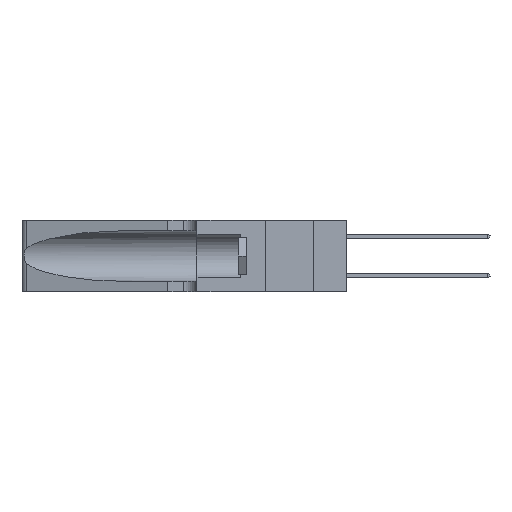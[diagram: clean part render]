
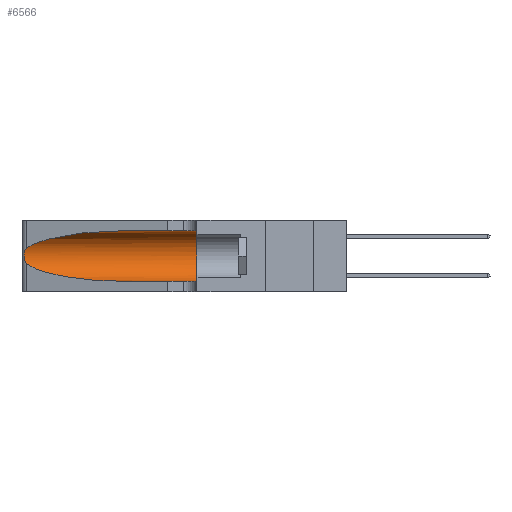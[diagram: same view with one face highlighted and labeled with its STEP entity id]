
A CAD part, left-side view. The second image highlights one B-rep face of the part: STEP entity #6566.
In plain terms, the highlighted cylindrical face has radius 3.308 mm (diameter 6.617 mm), a partial arc.
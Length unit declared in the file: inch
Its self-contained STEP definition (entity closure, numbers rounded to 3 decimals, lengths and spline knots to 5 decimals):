
#51 = VERTEX_POINT ( 'NONE', #33860 ) ;
#889 =( BOUNDED_CURVE ( )  B_SPLINE_CURVE ( 3, ( #27902, #6060, #30596, #14412 ),
 .UNSPECIFIED., .F., .F. ) 
 B_SPLINE_CURVE_WITH_KNOTS ( ( 4, 4 ),
 ( 3.44316, 4.71239 ),
 .UNSPECIFIED. ) 
 CURVE ( )  GEOMETRIC_REPRESENTATION_ITEM ( )  RATIONAL_B_SPLINE_CURVE ( ( 1., 0.87, 0.87, 1. ) ) 
 REPRESENTATION_ITEM ( '' )  );
#1834 = CARTESIAN_POINT ( 'NONE',  ( 0.1305, 0.35, 0.185 ) ) ;
#2090 = VERTEX_POINT ( 'NONE', #12327 ) ;
#2683 = CARTESIAN_POINT ( 'NONE',  ( 0.25789, 1.23486, 0.15765 ) ) ;
#3018 = VERTEX_POINT ( 'NONE', #10721 ) ;
#3440 = AXIS2_PLACEMENT_3D ( 'NONE', #1834, #20915, #4614 ) ;
#4614 = DIRECTION ( 'NONE',  ( 0., 0., 1. ) ) ;
#4886 = VERTEX_POINT ( 'NONE', #28967 ) ;
#4904 = DIRECTION ( 'NONE',  ( 0., -1., 0. ) ) ;
#5040 = CARTESIAN_POINT ( 'NONE',  ( 0.1305, 1.61858, 0.185 ) ) ;
#5468 = CARTESIAN_POINT ( 'NONE',  ( 0.25555, 1.22993, 0.14849 ) ) ;
#5615 = ORIENTED_EDGE ( 'NONE', *, *, #15021, .F. ) ;
#6060 = CARTESIAN_POINT ( 'NONE',  ( 0.2373, 1.15595, 0.08982 ) ) ;
#6566 = ADVANCED_FACE ( 'NONE', ( #17238 ), #14686, .F. ) ;
#6837 = VECTOR ( 'NONE', #8115, 39.37008 ) ;
#8083 = CARTESIAN_POINT ( 'NONE',  ( 0.25487, 1.22718, 0.22369 ) ) ;
#8115 = DIRECTION ( 'NONE',  ( 0., -1., 0. ) ) ;
#9631 = VERTEX_POINT ( 'NONE', #31602 ) ;
#9873 = EDGE_LOOP ( 'NONE', ( #21720, #22573, #23877, #31909, #11131, #5615 ) ) ;
#10218 = CARTESIAN_POINT ( 'NONE',  ( 0.1305, 0.72297, 0.31525 ) ) ;
#10361 = EDGE_CURVE ( 'NONE', #28154, #51, #12410, .T. ) ;
#10628 = CARTESIAN_POINT ( 'NONE',  ( 0.1305, 1.61858, 0.31525 ) ) ;
#10721 = CARTESIAN_POINT ( 'NONE',  ( 0.25487, 1.22718, 0.14631 ) ) ;
#10815 = CARTESIAN_POINT ( 'NONE',  ( 0.25787, 1.23484, 0.2124 ) ) ;
#11131 = ORIENTED_EDGE ( 'NONE', *, *, #10361, .F. ) ;
#11359 = LINE ( 'NONE', #10628, #32130 ) ;
#12327 = CARTESIAN_POINT ( 'NONE',  ( 0.25487, 1.22718, 0.22369 ) ) ;
#12410 = CIRCLE ( 'NONE', #3440, 0.13025 ) ;
#12768 = AXIS2_PLACEMENT_3D ( 'NONE', #5040, #4904, #24065 ) ;
#13270 = LINE ( 'NONE', #16354, #6837 ) ;
#13578 = CARTESIAN_POINT ( 'NONE',  ( 0.26018, 1.23835, 0.19895 ) ) ;
#13688 =( BOUNDED_CURVE ( )  B_SPLINE_CURVE ( 3, ( #10218, #26485, #15722, #34606 ),
 .UNSPECIFIED., .F., .F. ) 
 B_SPLINE_CURVE_WITH_KNOTS ( ( 4, 4 ),
 ( 1.5708, 2.84003 ),
 .UNSPECIFIED. ) 
 CURVE ( )  GEOMETRIC_REPRESENTATION_ITEM ( )  RATIONAL_B_SPLINE_CURVE ( ( 1., 0.87, 0.87, 1. ) ) 
 REPRESENTATION_ITEM ( '' )  );
#14412 = CARTESIAN_POINT ( 'NONE',  ( 0.1305, 0.72297, 0.05475 ) ) ;
#14686 = CYLINDRICAL_SURFACE ( 'NONE', #12768, 0.13025 ) ;
#15021 = EDGE_CURVE ( 'NONE', #4886, #28154, #11359, .T. ) ;
#15722 = CARTESIAN_POINT ( 'NONE',  ( 0.2373, 1.15595, 0.28018 ) ) ;
#16319 = CARTESIAN_POINT ( 'NONE',  ( 0.26075, 1.23896, 0.178 ) ) ;
#16354 = CARTESIAN_POINT ( 'NONE',  ( 0.1305, 1.61858, 0.05475 ) ) ;
#17238 = FACE_OUTER_BOUND ( 'NONE', #9873, .T. ) ;
#18956 = DIRECTION ( 'NONE',  ( 0., -1., 0. ) ) ;
#19032 = CARTESIAN_POINT ( 'NONE',  ( 0.25856, 1.23593, 0.16098 ) ) ;
#20915 = DIRECTION ( 'NONE',  ( 0., 1., 0. ) ) ;
#21720 = ORIENTED_EDGE ( 'NONE', *, *, #22995, .T. ) ;
#21727 = CARTESIAN_POINT ( 'NONE',  ( 0.25639, 1.23186, 0.15144 ) ) ;
#22468 = EDGE_CURVE ( 'NONE', #9631, #51, #13270, .T. ) ;
#22573 = ORIENTED_EDGE ( 'NONE', *, *, #35141, .T. ) ;
#22995 = EDGE_CURVE ( 'NONE', #4886, #2090, #13688, .T. ) ;
#23657 = B_SPLINE_CURVE_WITH_KNOTS ( 'NONE', 3,
 ( #8083, #24362, #27089, #10815, #29769, #13578, #32496, #16319, #35196, #19032, #2683, #21727, #5468, #24481 ),
 .UNSPECIFIED., .F., .F.,
 ( 4, 2, 2, 2, 2, 2, 4 ),
 ( 0., 0.00027, 0.00053, 0.00107, 0.0016, 0.00187, 0.00214 ),
 .UNSPECIFIED. ) ;
#23877 = ORIENTED_EDGE ( 'NONE', *, *, #32261, .T. ) ;
#24065 = DIRECTION ( 'NONE',  ( 0., 0., -1. ) ) ;
#24089 = CARTESIAN_POINT ( 'NONE',  ( 0.1305, 0.35, 0.31525 ) ) ;
#24362 = CARTESIAN_POINT ( 'NONE',  ( 0.25555, 1.22994, 0.2215 ) ) ;
#24481 = CARTESIAN_POINT ( 'NONE',  ( 0.25487, 1.22718, 0.14631 ) ) ;
#26485 = CARTESIAN_POINT ( 'NONE',  ( 0.18966, 0.96281, 0.31525 ) ) ;
#27089 = CARTESIAN_POINT ( 'NONE',  ( 0.25639, 1.23184, 0.21858 ) ) ;
#27902 = CARTESIAN_POINT ( 'NONE',  ( 0.25487, 1.22718, 0.14631 ) ) ;
#28154 = VERTEX_POINT ( 'NONE', #24089 ) ;
#28967 = CARTESIAN_POINT ( 'NONE',  ( 0.1305, 0.72297, 0.31525 ) ) ;
#29769 = CARTESIAN_POINT ( 'NONE',  ( 0.25854, 1.2359, 0.20912 ) ) ;
#30596 = CARTESIAN_POINT ( 'NONE',  ( 0.18966, 0.96281, 0.05475 ) ) ;
#31602 = CARTESIAN_POINT ( 'NONE',  ( 0.1305, 0.72297, 0.05475 ) ) ;
#31909 = ORIENTED_EDGE ( 'NONE', *, *, #22468, .T. ) ;
#32130 = VECTOR ( 'NONE', #18956, 39.37008 ) ;
#32261 = EDGE_CURVE ( 'NONE', #3018, #9631, #889, .T. ) ;
#32496 = CARTESIAN_POINT ( 'NONE',  ( 0.26075, 1.23896, 0.19203 ) ) ;
#33860 = CARTESIAN_POINT ( 'NONE',  ( 0.1305, 0.35, 0.05475 ) ) ;
#34606 = CARTESIAN_POINT ( 'NONE',  ( 0.25487, 1.22718, 0.22369 ) ) ;
#35141 = EDGE_CURVE ( 'NONE', #2090, #3018, #23657, .T. ) ;
#35196 = CARTESIAN_POINT ( 'NONE',  ( 0.26017, 1.23833, 0.17102 ) ) ;
